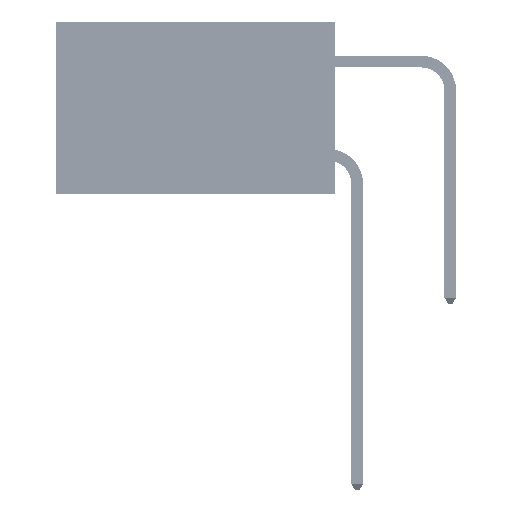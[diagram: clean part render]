
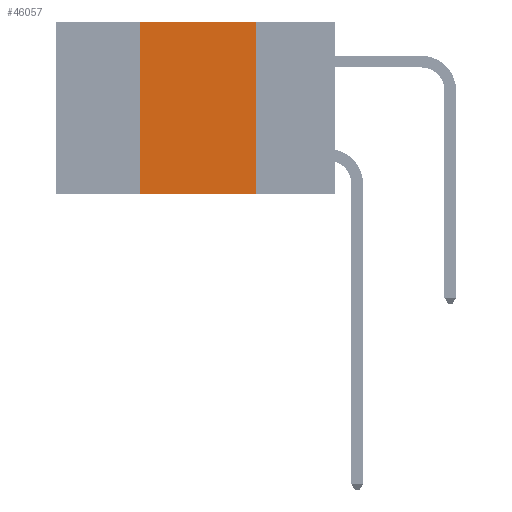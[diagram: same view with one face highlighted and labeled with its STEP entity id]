
A CAD part, left-side view. The second image highlights one B-rep face of the part: STEP entity #46057.
In plain terms, the highlighted planar face has unit normal (-1, 0, 0).
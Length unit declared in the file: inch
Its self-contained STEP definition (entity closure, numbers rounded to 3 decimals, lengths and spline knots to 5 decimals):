
#1760 = VECTOR ( 'NONE', #13526, 39.37008 ) ;
#2307 = PLANE ( 'NONE',  #24054 ) ;
#2492 = VECTOR ( 'NONE', #19840, 39.37008 ) ;
#6878 = CARTESIAN_POINT ( 'NONE',  ( 0., 0.17, -0.37 ) ) ;
#7613 = DIRECTION ( 'NONE',  ( 0., -1., 0. ) ) ;
#8796 = CARTESIAN_POINT ( 'NONE',  ( 0., 0.42, -0.37 ) ) ;
#11728 = VECTOR ( 'NONE', #7613, 39.37008 ) ;
#12072 = EDGE_CURVE ( 'NONE', #41812, #37818, #17039, .T. ) ;
#12547 = DIRECTION ( 'NONE',  ( 0., 0., 1. ) ) ;
#13526 = DIRECTION ( 'NONE',  ( 0., -1., 0. ) ) ;
#14323 = DIRECTION ( 'NONE',  ( 1., 0., 0. ) ) ;
#15550 = EDGE_CURVE ( 'NONE', #23285, #43616, #37102, .T. ) ;
#17039 = LINE ( 'NONE', #51787, #2492 ) ;
#17059 = CARTESIAN_POINT ( 'NONE',  ( 0., 0.6, -0.37 ) ) ;
#19840 = DIRECTION ( 'NONE',  ( 0., 0., -1. ) ) ;
#20060 = VECTOR ( 'NONE', #12547, 39.37008 ) ;
#20470 = CARTESIAN_POINT ( 'NONE',  ( 0., 0.42, 0. ) ) ;
#22445 = LINE ( 'NONE', #39205, #11728 ) ;
#23285 = VERTEX_POINT ( 'NONE', #8796 ) ;
#24054 = AXIS2_PLACEMENT_3D ( 'NONE', #46609, #14323, #30555 ) ;
#30555 = DIRECTION ( 'NONE',  ( 0., 0., -1. ) ) ;
#34283 = FACE_OUTER_BOUND ( 'NONE', #43998, .T. ) ;
#36497 = ORIENTED_EDGE ( 'NONE', *, *, #12072, .F. ) ;
#36683 = ORIENTED_EDGE ( 'NONE', *, *, #48464, .T. ) ;
#37102 = LINE ( 'NONE', #20470, #20060 ) ;
#37374 = CARTESIAN_POINT ( 'NONE',  ( 0., 0.17, 0. ) ) ;
#37818 = VERTEX_POINT ( 'NONE', #6878 ) ;
#39205 = CARTESIAN_POINT ( 'NONE',  ( 0., 0.6, 0. ) ) ;
#41812 = VERTEX_POINT ( 'NONE', #37374 ) ;
#43616 = VERTEX_POINT ( 'NONE', #43702 ) ;
#43702 = CARTESIAN_POINT ( 'NONE',  ( 0., 0.42, 0. ) ) ;
#43998 = EDGE_LOOP ( 'NONE', ( #36497, #44555, #51874, #36683 ) ) ;
#44555 = ORIENTED_EDGE ( 'NONE', *, *, #44716, .F. ) ;
#44716 = EDGE_CURVE ( 'NONE', #43616, #41812, #22445, .T. ) ;
#45959 = LINE ( 'NONE', #17059, #1760 ) ;
#46057 = ADVANCED_FACE ( 'NONE', ( #34283 ), #2307, .F. ) ;
#46609 = CARTESIAN_POINT ( 'NONE',  ( 0., 0.6, 0. ) ) ;
#48464 = EDGE_CURVE ( 'NONE', #23285, #37818, #45959, .T. ) ;
#51787 = CARTESIAN_POINT ( 'NONE',  ( 0., 0.17, 0. ) ) ;
#51874 = ORIENTED_EDGE ( 'NONE', *, *, #15550, .F. ) ;
